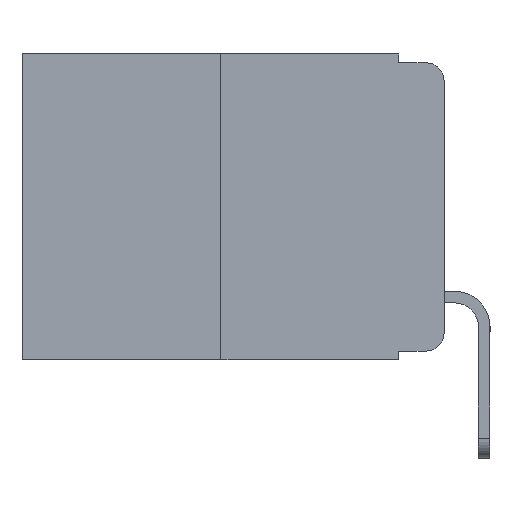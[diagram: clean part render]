
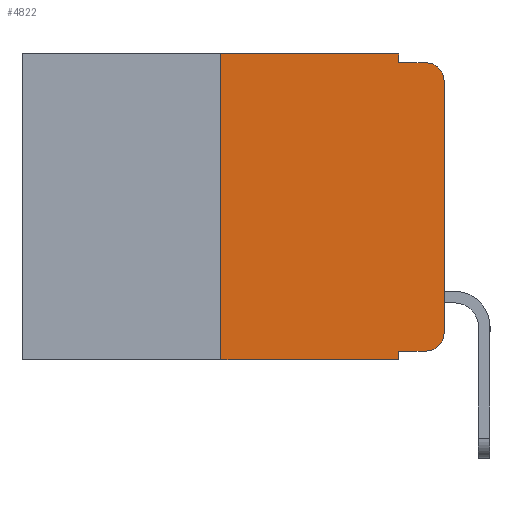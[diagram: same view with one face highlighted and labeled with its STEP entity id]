
A CAD part, left-side view. The second image highlights one B-rep face of the part: STEP entity #4822.
In plain terms, the highlighted planar face has unit normal (-1, 0, 0).
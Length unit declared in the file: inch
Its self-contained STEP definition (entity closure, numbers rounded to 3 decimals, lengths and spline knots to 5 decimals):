
#16 = ORIENTED_EDGE ( 'NONE', *, *, #11212, .T. ) ;
#150 = ORIENTED_EDGE ( 'NONE', *, *, #11243, .T. ) ;
#202 = DIRECTION ( 'NONE',  ( 0., 0., -1. ) ) ;
#320 = CARTESIAN_POINT ( 'NONE',  ( 0., 0.051, -0.333 ) ) ;
#489 = LINE ( 'NONE', #1160, #4982 ) ;
#508 = PLANE ( 'NONE',  #1002 ) ;
#768 = VECTOR ( 'NONE', #11550, 39.37008 ) ;
#785 = DIRECTION ( 'NONE',  ( 0., 0., 1. ) ) ;
#829 = LINE ( 'NONE', #11232, #7955 ) ;
#844 = LINE ( 'NONE', #1834, #8429 ) ;
#1002 = AXIS2_PLACEMENT_3D ( 'NONE', #2818, #10742, #10371 ) ;
#1160 = CARTESIAN_POINT ( 'NONE',  ( 0., 0.25, 0. ) ) ;
#1379 = DIRECTION ( 'NONE',  ( -1., 0., 0. ) ) ;
#1422 = CARTESIAN_POINT ( 'NONE',  ( 0., 0.051, -0.01 ) ) ;
#1726 = VERTEX_POINT ( 'NONE', #10902 ) ;
#1812 = VECTOR ( 'NONE', #5502, 39.37008 ) ;
#1834 = CARTESIAN_POINT ( 'NONE',  ( 0., 0., 0. ) ) ;
#1949 = CARTESIAN_POINT ( 'NONE',  ( 0., 0.051, -0.343 ) ) ;
#1962 = CARTESIAN_POINT ( 'NONE',  ( 0., 0.02, -0.333 ) ) ;
#2461 = VECTOR ( 'NONE', #11206, 39.37008 ) ;
#2512 = CARTESIAN_POINT ( 'NONE',  ( 0., 0.02, -0.313 ) ) ;
#2818 = CARTESIAN_POINT ( 'NONE',  ( 0., 0.473, 0. ) ) ;
#2937 = VECTOR ( 'NONE', #202, 39.37008 ) ;
#3437 = VERTEX_POINT ( 'NONE', #9335 ) ;
#3507 = DIRECTION ( 'NONE',  ( 0., -1., 0. ) ) ;
#3519 = LINE ( 'NONE', #10810, #768 ) ;
#3560 = DIRECTION ( 'NONE',  ( 0., 0., -1. ) ) ;
#4118 = EDGE_CURVE ( 'NONE', #5515, #5783, #10870, .T. ) ;
#4529 = LINE ( 'NONE', #1422, #1812 ) ;
#4822 = ADVANCED_FACE ( 'NONE', ( #9985 ), #508, .F. ) ;
#4982 = VECTOR ( 'NONE', #9369, 39.37008 ) ;
#5396 = VERTEX_POINT ( 'NONE', #5789 ) ;
#5502 = DIRECTION ( 'NONE',  ( 0., -1., 0. ) ) ;
#5515 = VERTEX_POINT ( 'NONE', #7272 ) ;
#5607 = VERTEX_POINT ( 'NONE', #6059 ) ;
#5756 = VERTEX_POINT ( 'NONE', #9794 ) ;
#5783 = VERTEX_POINT ( 'NONE', #1949 ) ;
#5785 = AXIS2_PLACEMENT_3D ( 'NONE', #2512, #8677, #3560 ) ;
#5789 = CARTESIAN_POINT ( 'NONE',  ( 0., 0., -0.313 ) ) ;
#6059 = CARTESIAN_POINT ( 'NONE',  ( 0., 0.02, -0.01 ) ) ;
#6204 = LINE ( 'NONE', #11076, #10215 ) ;
#6446 = DIRECTION ( 'NONE',  ( 0., 0., -1. ) ) ;
#6451 = CIRCLE ( 'NONE', #5785, 0.02 ) ;
#6459 = CARTESIAN_POINT ( 'NONE',  ( 0., 0.473, -0.343 ) ) ;
#6974 = CARTESIAN_POINT ( 'NONE',  ( 0., 0.051, 0. ) ) ;
#7061 = CARTESIAN_POINT ( 'NONE',  ( 0., 0.02, -0.03 ) ) ;
#7272 = CARTESIAN_POINT ( 'NONE',  ( 0., 0.25, -0.343 ) ) ;
#7799 = EDGE_CURVE ( 'NONE', #3437, #5756, #3519, .T. ) ;
#7865 = DIRECTION ( 'NONE',  ( 0., 0., -1. ) ) ;
#7955 = VECTOR ( 'NONE', #6446, 39.37008 ) ;
#8429 = VECTOR ( 'NONE', #785, 39.37008 ) ;
#8677 = DIRECTION ( 'NONE',  ( -1., 0., 0. ) ) ;
#9133 = VERTEX_POINT ( 'NONE', #1962 ) ;
#9159 = ORIENTED_EDGE ( 'NONE', *, *, #9999, .T. ) ;
#9167 = ORIENTED_EDGE ( 'NONE', *, *, #10391, .T. ) ;
#9177 = ORIENTED_EDGE ( 'NONE', *, *, #10430, .F. ) ;
#9178 = ORIENTED_EDGE ( 'NONE', *, *, #10504, .F. ) ;
#9188 = ORIENTED_EDGE ( 'NONE', *, *, #7799, .F. ) ;
#9213 = ORIENTED_EDGE ( 'NONE', *, *, #11107, .F. ) ;
#9277 = ORIENTED_EDGE ( 'NONE', *, *, #4118, .T. ) ;
#9295 = AXIS2_PLACEMENT_3D ( 'NONE', #7061, #1379, #7865 ) ;
#9335 = CARTESIAN_POINT ( 'NONE',  ( 0., 0.25, 0. ) ) ;
#9339 = LINE ( 'NONE', #6974, #2937 ) ;
#9343 = ORIENTED_EDGE ( 'NONE', *, *, #11141, .F. ) ;
#9369 = DIRECTION ( 'NONE',  ( 0., 0., 1. ) ) ;
#9457 = CARTESIAN_POINT ( 'NONE',  ( 0., 0., -0.03 ) ) ;
#9725 = VERTEX_POINT ( 'NONE', #320 ) ;
#9794 = CARTESIAN_POINT ( 'NONE',  ( 0., 0.051, 0. ) ) ;
#9985 = FACE_OUTER_BOUND ( 'NONE', #11238, .T. ) ;
#9999 = EDGE_CURVE ( 'NONE', #5396, #10375, #844, .T. ) ;
#10215 = VECTOR ( 'NONE', #3507, 39.37008 ) ;
#10371 = DIRECTION ( 'NONE',  ( 0., 0., -1. ) ) ;
#10375 = VERTEX_POINT ( 'NONE', #9457 ) ;
#10391 = EDGE_CURVE ( 'NONE', #10375, #5607, #11334, .T. ) ;
#10430 = EDGE_CURVE ( 'NONE', #1726, #5607, #4529, .T. ) ;
#10504 = EDGE_CURVE ( 'NONE', #5756, #1726, #829, .T. ) ;
#10742 = DIRECTION ( 'NONE',  ( 1., 0., 0. ) ) ;
#10810 = CARTESIAN_POINT ( 'NONE',  ( 0., 0.473, 0. ) ) ;
#10870 = LINE ( 'NONE', #6459, #2461 ) ;
#10902 = CARTESIAN_POINT ( 'NONE',  ( 0., 0.051, -0.01 ) ) ;
#11076 = CARTESIAN_POINT ( 'NONE',  ( 0., 0.051, -0.333 ) ) ;
#11107 = EDGE_CURVE ( 'NONE', #5515, #3437, #489, .T. ) ;
#11141 = EDGE_CURVE ( 'NONE', #9725, #5783, #9339, .T. ) ;
#11206 = DIRECTION ( 'NONE',  ( 0., -1., 0. ) ) ;
#11212 = EDGE_CURVE ( 'NONE', #9725, #9133, #6204, .T. ) ;
#11232 = CARTESIAN_POINT ( 'NONE',  ( 0., 0.051, 0. ) ) ;
#11238 = EDGE_LOOP ( 'NONE', ( #9159, #9167, #9177, #9178, #9188, #9213, #9277, #9343, #16, #150 ) ) ;
#11243 = EDGE_CURVE ( 'NONE', #9133, #5396, #6451, .T. ) ;
#11334 = CIRCLE ( 'NONE', #9295, 0.02 ) ;
#11550 = DIRECTION ( 'NONE',  ( 0., -1., 0. ) ) ;
